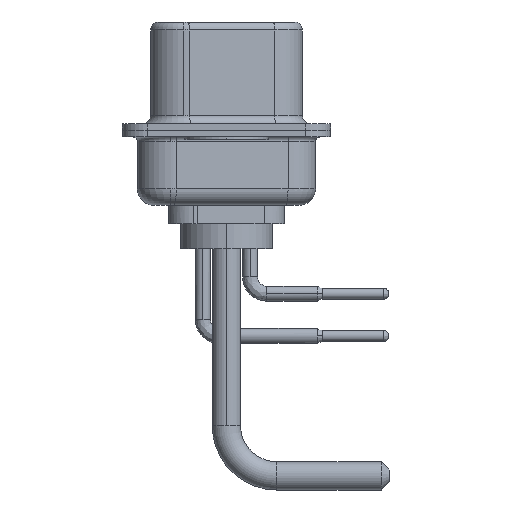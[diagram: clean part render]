
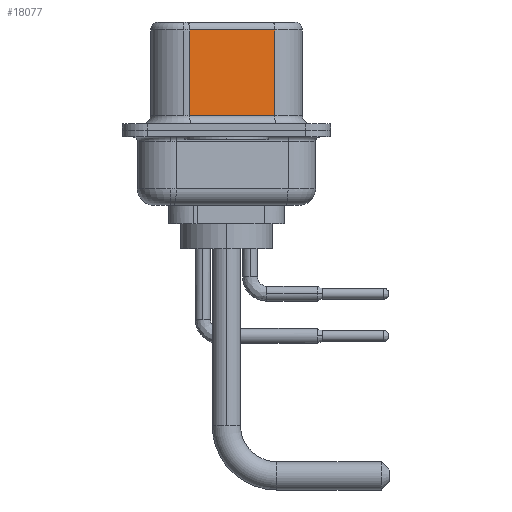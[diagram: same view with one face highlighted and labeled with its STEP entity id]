
A CAD part, left-side view. The second image highlights one B-rep face of the part: STEP entity #18077.
In plain terms, the highlighted planar face has unit normal (-0.985, -0.174, 0).
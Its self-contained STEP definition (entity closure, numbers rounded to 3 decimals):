
#144 = DIRECTION ( 'NONE',  ( 0.985, 0.174, 0. ) ) ;
#1757 = VERTEX_POINT ( 'NONE', #6461 ) ;
#2340 = CARTESIAN_POINT ( 'NONE',  ( 3.68, 2.203, 0.9 ) ) ;
#3613 = FACE_OUTER_BOUND ( 'NONE', #17672, .T. ) ;
#4696 = VERTEX_POINT ( 'NONE', #2340 ) ;
#5175 = VECTOR ( 'NONE', #11172, 1000. ) ;
#5398 = AXIS2_PLACEMENT_3D ( 'NONE', #13249, #144, #5647 ) ;
#5647 = DIRECTION ( 'NONE',  ( -0.174, 0.985, 0. ) ) ;
#5876 = CARTESIAN_POINT ( 'NONE',  ( 3.68, 2.203, 6.02 ) ) ;
#5886 = PLANE ( 'NONE',  #5398 ) ;
#6461 = CARTESIAN_POINT ( 'NONE',  ( 4.58, -2.897, 6.02 ) ) ;
#7011 = EDGE_CURVE ( 'NONE', #9189, #4696, #14587, .T. ) ;
#8041 = CARTESIAN_POINT ( 'NONE',  ( 4.58, -2.897, 6.02 ) ) ;
#8897 = ORIENTED_EDGE ( 'NONE', *, *, #9366, .T. ) ;
#9189 = VERTEX_POINT ( 'NONE', #5876 ) ;
#9245 = LINE ( 'NONE', #10810, #5175 ) ;
#9366 = EDGE_CURVE ( 'NONE', #4696, #16408, #9245, .T. ) ;
#10810 = CARTESIAN_POINT ( 'NONE',  ( 4.58, -2.897, 0.9 ) ) ;
#11172 = DIRECTION ( 'NONE',  ( 0.174, -0.985, 0. ) ) ;
#11204 = DIRECTION ( 'NONE',  ( 0., 0., -1. ) ) ;
#12944 = DIRECTION ( 'NONE',  ( 0., 0., -1. ) ) ;
#12968 = VECTOR ( 'NONE', #11204, 1000. ) ;
#13002 = ORIENTED_EDGE ( 'NONE', *, *, #14267, .F. ) ;
#13249 = CARTESIAN_POINT ( 'NONE',  ( 4.58, -2.897, 6.52 ) ) ;
#13587 = LINE ( 'NONE', #8041, #15396 ) ;
#14267 = EDGE_CURVE ( 'NONE', #1757, #16408, #16569, .T. ) ;
#14587 = LINE ( 'NONE', #20382, #12968 ) ;
#14725 = VECTOR ( 'NONE', #12944, 1000. ) ;
#15395 = DIRECTION ( 'NONE',  ( -0.174, 0.985, 0. ) ) ;
#15396 = VECTOR ( 'NONE', #15395, 1000. ) ;
#16022 = CARTESIAN_POINT ( 'NONE',  ( 4.58, -2.897, 0.9 ) ) ;
#16408 = VERTEX_POINT ( 'NONE', #16022 ) ;
#16417 = ORIENTED_EDGE ( 'NONE', *, *, #17893, .T. ) ;
#16569 = LINE ( 'NONE', #16681, #14725 ) ;
#16681 = CARTESIAN_POINT ( 'NONE',  ( 4.58, -2.897, 6.52 ) ) ;
#17672 = EDGE_LOOP ( 'NONE', ( #13002, #16417, #18370, #8897 ) ) ;
#17893 = EDGE_CURVE ( 'NONE', #1757, #9189, #13587, .T. ) ;
#18077 = ADVANCED_FACE ( 'NONE', ( #3613 ), #5886, .F. ) ;
#18370 = ORIENTED_EDGE ( 'NONE', *, *, #7011, .T. ) ;
#20382 = CARTESIAN_POINT ( 'NONE',  ( 3.68, 2.203, 6.52 ) ) ;
